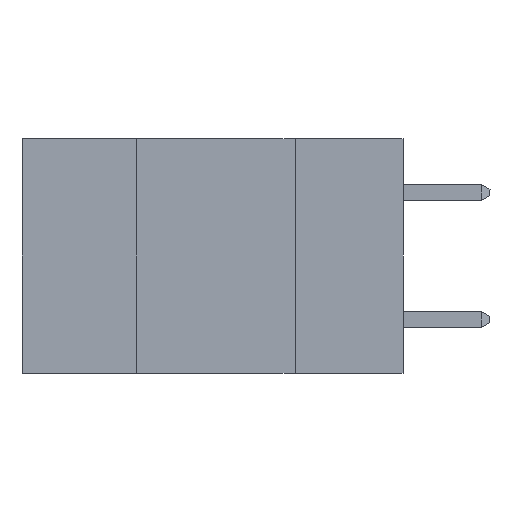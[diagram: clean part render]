
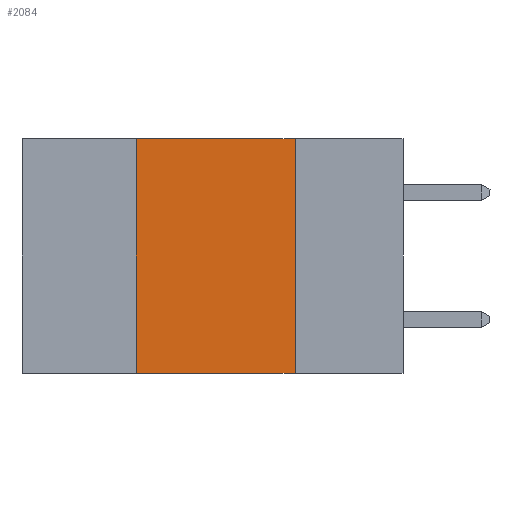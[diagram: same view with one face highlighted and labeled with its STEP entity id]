
A CAD part, left-side view. The second image highlights one B-rep face of the part: STEP entity #2084.
In plain terms, the highlighted planar face has unit normal (-1, 0, 0).
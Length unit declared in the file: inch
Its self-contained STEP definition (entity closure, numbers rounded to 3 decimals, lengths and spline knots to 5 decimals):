
#156 = VERTEX_POINT ( 'NONE', #5746 ) ;
#463 = VECTOR ( 'NONE', #2105, 39.37008 ) ;
#856 = LINE ( 'NONE', #10236, #7384 ) ;
#1702 = DIRECTION ( 'NONE',  ( 0., 0., -1. ) ) ;
#2084 = ADVANCED_FACE ( 'NONE', ( #8629 ), #5979, .F. ) ;
#2105 = DIRECTION ( 'NONE',  ( 0., 0., 1. ) ) ;
#2547 = CARTESIAN_POINT ( 'NONE',  ( 0., 0.6, 0. ) ) ;
#2901 = ORIENTED_EDGE ( 'NONE', *, *, #5977, .F. ) ;
#3048 = CARTESIAN_POINT ( 'NONE',  ( 0., 0.6, -0.37 ) ) ;
#3118 = EDGE_CURVE ( 'NONE', #4998, #5319, #5567, .T. ) ;
#3488 = VECTOR ( 'NONE', #10082, 39.37008 ) ;
#3706 = EDGE_LOOP ( 'NONE', ( #2901, #9600, #5444, #8471 ) ) ;
#3907 = DIRECTION ( 'NONE',  ( 0., -1., 0. ) ) ;
#4846 = EDGE_CURVE ( 'NONE', #4998, #5951, #7275, .T. ) ;
#4998 = VERTEX_POINT ( 'NONE', #10647 ) ;
#5242 = CARTESIAN_POINT ( 'NONE',  ( 0., 0.42, 0. ) ) ;
#5277 = DIRECTION ( 'NONE',  ( 0., 0., -1. ) ) ;
#5319 = VERTEX_POINT ( 'NONE', #8641 ) ;
#5444 = ORIENTED_EDGE ( 'NONE', *, *, #4846, .F. ) ;
#5567 = LINE ( 'NONE', #3048, #7821 ) ;
#5746 = CARTESIAN_POINT ( 'NONE',  ( 0., 0.17, 0. ) ) ;
#5951 = VERTEX_POINT ( 'NONE', #5242 ) ;
#5977 = EDGE_CURVE ( 'NONE', #156, #5319, #856, .T. ) ;
#5979 = PLANE ( 'NONE',  #8561 ) ;
#6345 = CARTESIAN_POINT ( 'NONE',  ( 0., 0.42, 0. ) ) ;
#6761 = CARTESIAN_POINT ( 'NONE',  ( 0., 0.6, 0. ) ) ;
#6824 = DIRECTION ( 'NONE',  ( 1., 0., 0. ) ) ;
#7036 = EDGE_CURVE ( 'NONE', #5951, #156, #8006, .T. ) ;
#7275 = LINE ( 'NONE', #6345, #463 ) ;
#7384 = VECTOR ( 'NONE', #5277, 39.37008 ) ;
#7821 = VECTOR ( 'NONE', #3907, 39.37008 ) ;
#8006 = LINE ( 'NONE', #6761, #3488 ) ;
#8471 = ORIENTED_EDGE ( 'NONE', *, *, #3118, .T. ) ;
#8561 = AXIS2_PLACEMENT_3D ( 'NONE', #2547, #6824, #1702 ) ;
#8629 = FACE_OUTER_BOUND ( 'NONE', #3706, .T. ) ;
#8641 = CARTESIAN_POINT ( 'NONE',  ( 0., 0.17, -0.37 ) ) ;
#9600 = ORIENTED_EDGE ( 'NONE', *, *, #7036, .F. ) ;
#10082 = DIRECTION ( 'NONE',  ( 0., -1., 0. ) ) ;
#10236 = CARTESIAN_POINT ( 'NONE',  ( 0., 0.17, 0. ) ) ;
#10647 = CARTESIAN_POINT ( 'NONE',  ( 0., 0.42, -0.37 ) ) ;
